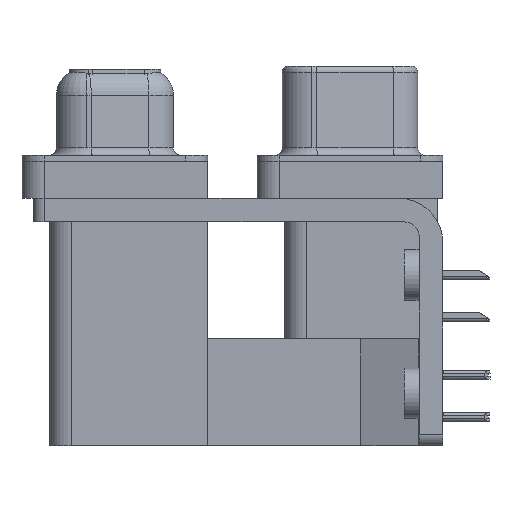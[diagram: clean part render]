
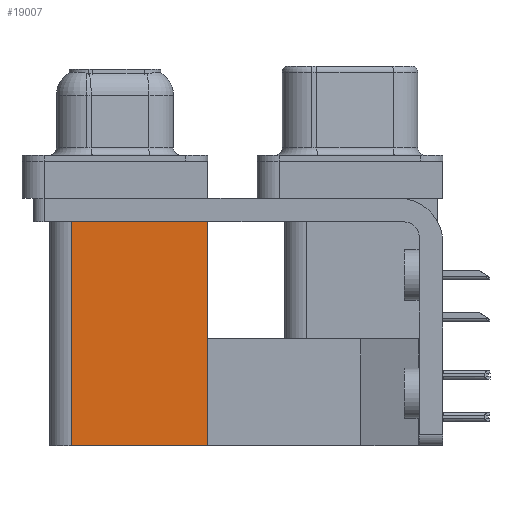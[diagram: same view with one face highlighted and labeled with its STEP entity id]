
A CAD part, left-side view. The second image highlights one B-rep face of the part: STEP entity #19007.
In plain terms, the highlighted planar face has unit normal (-1, 0, 0).
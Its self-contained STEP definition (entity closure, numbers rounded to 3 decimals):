
#399 = VECTOR ( 'NONE', #10492, 1000. ) ;
#726 = LINE ( 'NONE', #19144, #1116 ) ;
#1116 = VECTOR ( 'NONE', #31377, 1000. ) ;
#1214 = CARTESIAN_POINT ( 'NONE',  ( 3.79, 18.8, -2.5 ) ) ;
#3292 = DIRECTION ( 'NONE',  ( 0., 1., 0. ) ) ;
#4434 = LINE ( 'NONE', #13806, #7626 ) ;
#4997 = EDGE_CURVE ( 'NONE', #15738, #10717, #28443, .T. ) ;
#5025 = DIRECTION ( 'NONE',  ( 0., 0., 1. ) ) ;
#5588 = PLANE ( 'NONE',  #35598 ) ;
#7626 = VECTOR ( 'NONE', #5025, 1000. ) ;
#7990 = VERTEX_POINT ( 'NONE', #33215 ) ;
#9710 = LINE ( 'NONE', #16097, #399 ) ;
#10492 = DIRECTION ( 'NONE',  ( 0., 1., 0. ) ) ;
#10717 = VERTEX_POINT ( 'NONE', #1214 ) ;
#12456 = CARTESIAN_POINT ( 'NONE',  ( 3.79, 9.6, -2.5 ) ) ;
#13198 = CARTESIAN_POINT ( 'NONE',  ( 3.79, 9.6, -2.5 ) ) ;
#13444 = DIRECTION ( 'NONE',  ( 0., 1., 0. ) ) ;
#13806 = CARTESIAN_POINT ( 'NONE',  ( 3.79, 18.8, -19.2 ) ) ;
#14078 = ORIENTED_EDGE ( 'NONE', *, *, #25227, .F. ) ;
#15738 = VERTEX_POINT ( 'NONE', #12456 ) ;
#16097 = CARTESIAN_POINT ( 'NONE',  ( 3.79, 9.6, -19.2 ) ) ;
#19007 = ADVANCED_FACE ( 'NONE', ( #25672 ), #5588, .F. ) ;
#19144 = CARTESIAN_POINT ( 'NONE',  ( 3.79, 9.6, -19.2 ) ) ;
#19145 = VERTEX_POINT ( 'NONE', #24220 ) ;
#20790 = CARTESIAN_POINT ( 'NONE',  ( 3.79, 9.6, -19.2 ) ) ;
#22089 = EDGE_CURVE ( 'NONE', #19145, #15738, #726, .T. ) ;
#23473 = VECTOR ( 'NONE', #3292, 1000. ) ;
#24220 = CARTESIAN_POINT ( 'NONE',  ( 3.79, 9.6, -19.2 ) ) ;
#25227 = EDGE_CURVE ( 'NONE', #7990, #10717, #4434, .T. ) ;
#25672 = FACE_OUTER_BOUND ( 'NONE', #39382, .T. ) ;
#26779 = ORIENTED_EDGE ( 'NONE', *, *, #35131, .F. ) ;
#28443 = LINE ( 'NONE', #13198, #23473 ) ;
#31377 = DIRECTION ( 'NONE',  ( 0., 0., 1. ) ) ;
#32945 = ORIENTED_EDGE ( 'NONE', *, *, #4997, .T. ) ;
#33215 = CARTESIAN_POINT ( 'NONE',  ( 3.79, 18.8, -19.2 ) ) ;
#35131 = EDGE_CURVE ( 'NONE', #19145, #7990, #9710, .T. ) ;
#35598 = AXIS2_PLACEMENT_3D ( 'NONE', #20790, #36049, #13444 ) ;
#36049 = DIRECTION ( 'NONE',  ( 1., 0., 0. ) ) ;
#38976 = ORIENTED_EDGE ( 'NONE', *, *, #22089, .T. ) ;
#39382 = EDGE_LOOP ( 'NONE', ( #32945, #14078, #26779, #38976 ) ) ;
